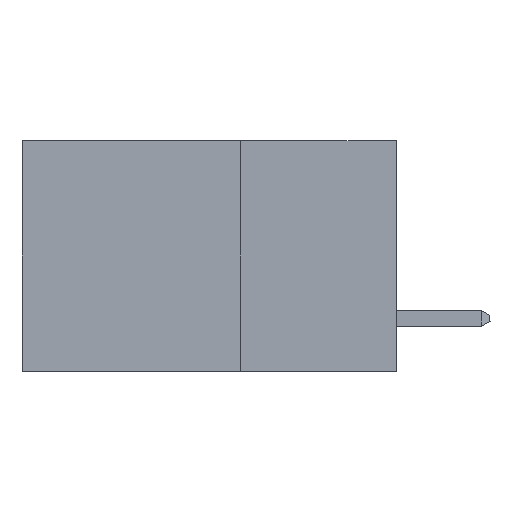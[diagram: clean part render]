
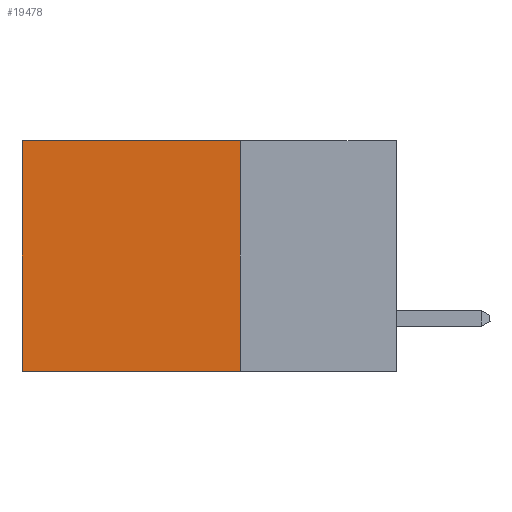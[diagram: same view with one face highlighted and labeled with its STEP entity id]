
A CAD part, left-side view. The second image highlights one B-rep face of the part: STEP entity #19478.
In plain terms, the highlighted planar face has unit normal (-1, 0, 0).
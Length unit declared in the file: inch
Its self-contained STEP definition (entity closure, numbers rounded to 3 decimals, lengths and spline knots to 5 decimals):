
#1718 = VERTEX_POINT ( 'NONE', #7924 ) ;
#1790 = DIRECTION ( 'NONE',  ( 0., 0., -1. ) ) ;
#1976 = LINE ( 'NONE', #10380, #15838 ) ;
#2068 = LINE ( 'NONE', #17784, #20036 ) ;
#3063 = VECTOR ( 'NONE', #22031, 39.37008 ) ;
#4650 = ORIENTED_EDGE ( 'NONE', *, *, #9020, .F. ) ;
#5302 = EDGE_CURVE ( 'NONE', #1718, #20207, #1976, .T. ) ;
#5625 = EDGE_LOOP ( 'NONE', ( #13274, #16080, #4650, #15674 ) ) ;
#7924 = CARTESIAN_POINT ( 'NONE',  ( 0.298, 0.25, 0. ) ) ;
#8342 = LINE ( 'NONE', #21901, #16961 ) ;
#8758 = FACE_OUTER_BOUND ( 'NONE', #5625, .T. ) ;
#8774 = PLANE ( 'NONE',  #15742 ) ;
#9020 = EDGE_CURVE ( 'NONE', #1718, #16710, #2068, .T. ) ;
#10380 = CARTESIAN_POINT ( 'NONE',  ( 0.298, 0.25, 0. ) ) ;
#10526 = EDGE_CURVE ( 'NONE', #20207, #19004, #21525, .T. ) ;
#11580 = CARTESIAN_POINT ( 'NONE',  ( 0.298, 0.25, -0.37 ) ) ;
#12233 = DIRECTION ( 'NONE',  ( 1., 0., 0. ) ) ;
#12632 = DIRECTION ( 'NONE',  ( 0., 0., -1. ) ) ;
#13274 = ORIENTED_EDGE ( 'NONE', *, *, #10526, .T. ) ;
#15674 = ORIENTED_EDGE ( 'NONE', *, *, #5302, .T. ) ;
#15742 = AXIS2_PLACEMENT_3D ( 'NONE', #22606, #12233, #1790 ) ;
#15838 = VECTOR ( 'NONE', #20769, 39.37008 ) ;
#16080 = ORIENTED_EDGE ( 'NONE', *, *, #18572, .F. ) ;
#16710 = VERTEX_POINT ( 'NONE', #11580 ) ;
#16961 = VECTOR ( 'NONE', #20166, 39.37008 ) ;
#17784 = CARTESIAN_POINT ( 'NONE',  ( 0.298, 0.25, 0. ) ) ;
#18572 = EDGE_CURVE ( 'NONE', #16710, #19004, #8342, .T. ) ;
#19004 = VERTEX_POINT ( 'NONE', #19607 ) ;
#19478 = ADVANCED_FACE ( 'NONE', ( #8758 ), #8774, .F. ) ;
#19607 = CARTESIAN_POINT ( 'NONE',  ( 0.298, 0.6, -0.37 ) ) ;
#19644 = CARTESIAN_POINT ( 'NONE',  ( 0.298, 0.6, 0. ) ) ;
#20036 = VECTOR ( 'NONE', #12632, 39.37008 ) ;
#20166 = DIRECTION ( 'NONE',  ( 0., 1., 0. ) ) ;
#20207 = VERTEX_POINT ( 'NONE', #19644 ) ;
#20282 = CARTESIAN_POINT ( 'NONE',  ( 0.298, 0.6, 0. ) ) ;
#20769 = DIRECTION ( 'NONE',  ( 0., 1., 0. ) ) ;
#21525 = LINE ( 'NONE', #20282, #3063 ) ;
#21901 = CARTESIAN_POINT ( 'NONE',  ( 0.298, 0.25, -0.37 ) ) ;
#22031 = DIRECTION ( 'NONE',  ( 0., 0., -1. ) ) ;
#22606 = CARTESIAN_POINT ( 'NONE',  ( 0.298, 0.25, 0. ) ) ;
